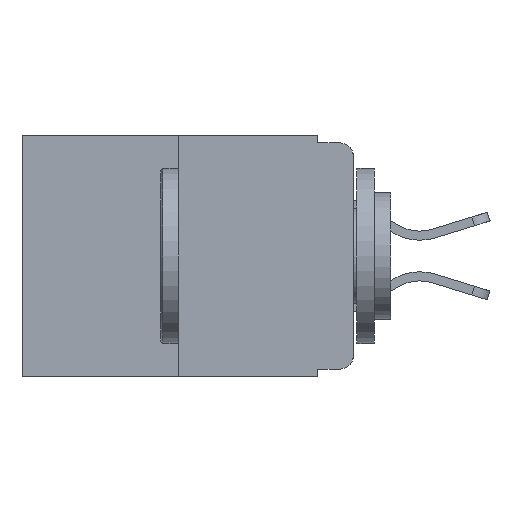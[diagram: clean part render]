
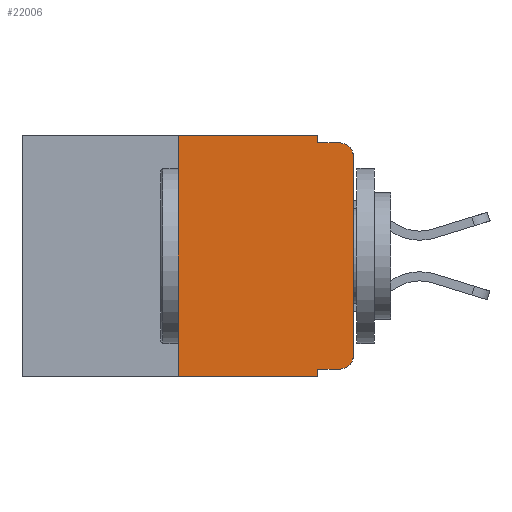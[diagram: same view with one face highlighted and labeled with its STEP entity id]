
A CAD part, left-side view. The second image highlights one B-rep face of the part: STEP entity #22006.
In plain terms, the highlighted planar face has unit normal (-1, 0, 0).
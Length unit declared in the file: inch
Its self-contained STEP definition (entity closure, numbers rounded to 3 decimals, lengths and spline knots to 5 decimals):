
#319 = VECTOR ( 'NONE', #12351, 39.37008 ) ;
#696 = VERTEX_POINT ( 'NONE', #9755 ) ;
#754 = ORIENTED_EDGE ( 'NONE', *, *, #15806, .T. ) ;
#1280 = CARTESIAN_POINT ( 'NONE',  ( 0., 0.25, -0.343 ) ) ;
#1621 = CIRCLE ( 'NONE', #13864, 0.02 ) ;
#1667 = VERTEX_POINT ( 'NONE', #7799 ) ;
#2011 = CARTESIAN_POINT ( 'NONE',  ( 0., 0.02, -0.01 ) ) ;
#2196 = FACE_OUTER_BOUND ( 'NONE', #10613, .T. ) ;
#2282 = CARTESIAN_POINT ( 'NONE',  ( 0., 0., -0.313 ) ) ;
#2748 = CARTESIAN_POINT ( 'NONE',  ( 0., 0., -0.03 ) ) ;
#2929 = VECTOR ( 'NONE', #6959, 39.37008 ) ;
#3150 = EDGE_CURVE ( 'NONE', #15531, #6140, #3423, .T. ) ;
#3317 = AXIS2_PLACEMENT_3D ( 'NONE', #4249, #6283, #22999 ) ;
#3423 = LINE ( 'NONE', #5725, #17408 ) ;
#3561 = VECTOR ( 'NONE', #14152, 39.37008 ) ;
#3703 = ORIENTED_EDGE ( 'NONE', *, *, #3150, .T. ) ;
#4030 = CARTESIAN_POINT ( 'NONE',  ( 0., 0.051, 0. ) ) ;
#4249 = CARTESIAN_POINT ( 'NONE',  ( 0., 0.473, 0. ) ) ;
#4384 = CARTESIAN_POINT ( 'NONE',  ( 0., 0.25, 0. ) ) ;
#4476 = CIRCLE ( 'NONE', #4498, 0.02 ) ;
#4498 = AXIS2_PLACEMENT_3D ( 'NONE', #15168, #25467, #13257 ) ;
#4565 = VERTEX_POINT ( 'NONE', #13283 ) ;
#5409 = CARTESIAN_POINT ( 'NONE',  ( 0., 0.051, -0.333 ) ) ;
#5725 = CARTESIAN_POINT ( 'NONE',  ( 0., 0., 0. ) ) ;
#6069 = EDGE_CURVE ( 'NONE', #17591, #4565, #19172, .T. ) ;
#6078 = LINE ( 'NONE', #4030, #319 ) ;
#6140 = VERTEX_POINT ( 'NONE', #2748 ) ;
#6220 = ORIENTED_EDGE ( 'NONE', *, *, #24280, .F. ) ;
#6230 = LINE ( 'NONE', #8821, #23614 ) ;
#6283 = DIRECTION ( 'NONE',  ( 1., 0., 0. ) ) ;
#6620 = DIRECTION ( 'NONE',  ( 0., -1., 0. ) ) ;
#6959 = DIRECTION ( 'NONE',  ( 0., 0., -1. ) ) ;
#7478 = ORIENTED_EDGE ( 'NONE', *, *, #24017, .T. ) ;
#7799 = CARTESIAN_POINT ( 'NONE',  ( 0., 0.051, 0. ) ) ;
#7848 = ORIENTED_EDGE ( 'NONE', *, *, #8079, .T. ) ;
#8079 = EDGE_CURVE ( 'NONE', #17591, #12748, #8397, .T. ) ;
#8397 = LINE ( 'NONE', #25400, #20645 ) ;
#8478 = EDGE_CURVE ( 'NONE', #17484, #15531, #4476, .T. ) ;
#8641 = LINE ( 'NONE', #25362, #26026 ) ;
#8684 = ORIENTED_EDGE ( 'NONE', *, *, #13117, .F. ) ;
#8821 = CARTESIAN_POINT ( 'NONE',  ( 0., 0.051, -0.01 ) ) ;
#8824 = DIRECTION ( 'NONE',  ( 0., 0., -1. ) ) ;
#8876 = DIRECTION ( 'NONE',  ( 0., 0., 1. ) ) ;
#9755 = CARTESIAN_POINT ( 'NONE',  ( 0., 0.051, -0.01 ) ) ;
#10536 = ORIENTED_EDGE ( 'NONE', *, *, #8478, .T. ) ;
#10613 = EDGE_LOOP ( 'NONE', ( #3703, #7478, #8684, #6220, #26106, #22304, #7848, #24869, #754, #10536 ) ) ;
#10829 = VERTEX_POINT ( 'NONE', #5409 ) ;
#11573 = CARTESIAN_POINT ( 'NONE',  ( 0., 0.051, -0.343 ) ) ;
#12351 = DIRECTION ( 'NONE',  ( 0., 0., -1. ) ) ;
#12510 = VECTOR ( 'NONE', #8876, 39.37008 ) ;
#12748 = VERTEX_POINT ( 'NONE', #11573 ) ;
#13117 = EDGE_CURVE ( 'NONE', #696, #16750, #6230, .T. ) ;
#13257 = DIRECTION ( 'NONE',  ( 0., 0., -1. ) ) ;
#13283 = CARTESIAN_POINT ( 'NONE',  ( 0., 0.25, 0. ) ) ;
#13864 = AXIS2_PLACEMENT_3D ( 'NONE', #25557, #19255, #8824 ) ;
#14152 = DIRECTION ( 'NONE',  ( 0., -1., 0. ) ) ;
#15168 = CARTESIAN_POINT ( 'NONE',  ( 0., 0.02, -0.313 ) ) ;
#15531 = VERTEX_POINT ( 'NONE', #2282 ) ;
#15806 = EDGE_CURVE ( 'NONE', #10829, #17484, #22117, .T. ) ;
#16750 = VERTEX_POINT ( 'NONE', #2011 ) ;
#16987 = DIRECTION ( 'NONE',  ( 0., -1., 0. ) ) ;
#17358 = LINE ( 'NONE', #25732, #2929 ) ;
#17408 = VECTOR ( 'NONE', #18319, 39.37008 ) ;
#17484 = VERTEX_POINT ( 'NONE', #19495 ) ;
#17591 = VERTEX_POINT ( 'NONE', #1280 ) ;
#18319 = DIRECTION ( 'NONE',  ( 0., 0., 1. ) ) ;
#19172 = LINE ( 'NONE', #4384, #12510 ) ;
#19255 = DIRECTION ( 'NONE',  ( -1., 0., 0. ) ) ;
#19495 = CARTESIAN_POINT ( 'NONE',  ( 0., 0.02, -0.333 ) ) ;
#20645 = VECTOR ( 'NONE', #6620, 39.37008 ) ;
#21518 = EDGE_CURVE ( 'NONE', #4565, #1667, #8641, .T. ) ;
#22006 = ADVANCED_FACE ( 'NONE', ( #2196 ), #25055, .F. ) ;
#22117 = LINE ( 'NONE', #26506, #3561 ) ;
#22304 = ORIENTED_EDGE ( 'NONE', *, *, #6069, .F. ) ;
#22999 = DIRECTION ( 'NONE',  ( 0., 0., -1. ) ) ;
#23584 = EDGE_CURVE ( 'NONE', #10829, #12748, #17358, .T. ) ;
#23614 = VECTOR ( 'NONE', #24876, 39.37008 ) ;
#24017 = EDGE_CURVE ( 'NONE', #6140, #16750, #1621, .T. ) ;
#24280 = EDGE_CURVE ( 'NONE', #1667, #696, #6078, .T. ) ;
#24869 = ORIENTED_EDGE ( 'NONE', *, *, #23584, .F. ) ;
#24876 = DIRECTION ( 'NONE',  ( 0., -1., 0. ) ) ;
#25055 = PLANE ( 'NONE',  #3317 ) ;
#25362 = CARTESIAN_POINT ( 'NONE',  ( 0., 0.473, 0. ) ) ;
#25400 = CARTESIAN_POINT ( 'NONE',  ( 0., 0.473, -0.343 ) ) ;
#25467 = DIRECTION ( 'NONE',  ( -1., 0., 0. ) ) ;
#25557 = CARTESIAN_POINT ( 'NONE',  ( 0., 0.02, -0.03 ) ) ;
#25732 = CARTESIAN_POINT ( 'NONE',  ( 0., 0.051, 0. ) ) ;
#26026 = VECTOR ( 'NONE', #16987, 39.37008 ) ;
#26106 = ORIENTED_EDGE ( 'NONE', *, *, #21518, .F. ) ;
#26506 = CARTESIAN_POINT ( 'NONE',  ( 0., 0.051, -0.333 ) ) ;
